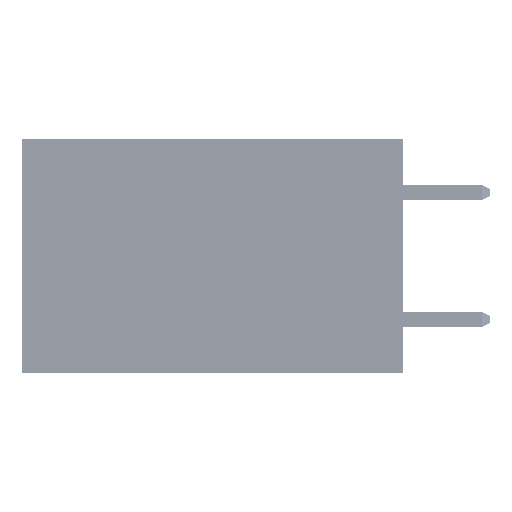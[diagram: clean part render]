
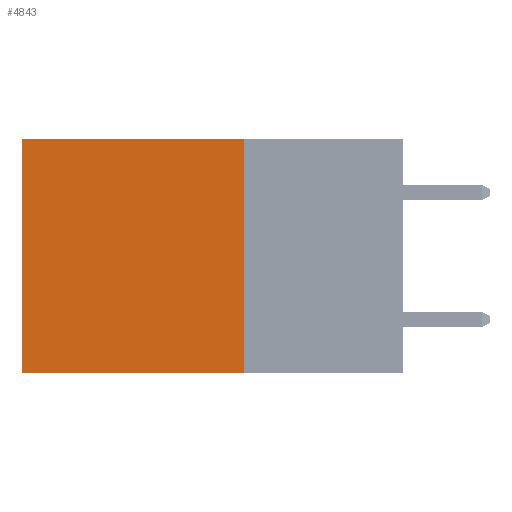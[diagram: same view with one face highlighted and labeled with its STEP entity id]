
A CAD part, left-side view. The second image highlights one B-rep face of the part: STEP entity #4843.
In plain terms, the highlighted planar face has unit normal (-1, 0, 0).
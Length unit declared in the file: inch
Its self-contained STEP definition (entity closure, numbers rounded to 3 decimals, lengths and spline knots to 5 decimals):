
#866 = ORIENTED_EDGE ( 'NONE', *, *, #38882, .F. ) ;
#1009 = CARTESIAN_POINT ( 'NONE',  ( 0.2875, 0.25, 0. ) ) ;
#1629 = CARTESIAN_POINT ( 'NONE',  ( 0.2875, 0.6, -0.37 ) ) ;
#2280 = ORIENTED_EDGE ( 'NONE', *, *, #23663, .F. ) ;
#3140 = VECTOR ( 'NONE', #40753, 39.37008 ) ;
#3284 = CARTESIAN_POINT ( 'NONE',  ( 0.2875, 0.25, 0. ) ) ;
#4843 = ADVANCED_FACE ( 'NONE', ( #8497 ), #8032, .F. ) ;
#6548 = VECTOR ( 'NONE', #10634, 39.37008 ) ;
#7323 = DIRECTION ( 'NONE',  ( 0., 0., -1. ) ) ;
#7784 = DIRECTION ( 'NONE',  ( 0., 0., -1. ) ) ;
#7798 = VECTOR ( 'NONE', #21353, 39.37008 ) ;
#8032 = PLANE ( 'NONE',  #33689 ) ;
#8497 = FACE_OUTER_BOUND ( 'NONE', #36221, .T. ) ;
#9017 = CARTESIAN_POINT ( 'NONE',  ( 0.2875, 0.25, 0. ) ) ;
#10634 = DIRECTION ( 'NONE',  ( 0., 1., 0. ) ) ;
#14505 = EDGE_CURVE ( 'NONE', #36444, #36766, #25422, .T. ) ;
#14585 = CARTESIAN_POINT ( 'NONE',  ( 0.2875, 0.6, 0. ) ) ;
#16165 = CARTESIAN_POINT ( 'NONE',  ( 0.2875, 0.25, 0. ) ) ;
#17541 = ORIENTED_EDGE ( 'NONE', *, *, #14505, .T. ) ;
#17640 = LINE ( 'NONE', #9017, #6548 ) ;
#18580 = VERTEX_POINT ( 'NONE', #16165 ) ;
#19528 = VERTEX_POINT ( 'NONE', #40727 ) ;
#21353 = DIRECTION ( 'NONE',  ( 0., 1., 0. ) ) ;
#23663 = EDGE_CURVE ( 'NONE', #19528, #36766, #36310, .T. ) ;
#25041 = LINE ( 'NONE', #3284, #3140 ) ;
#25422 = LINE ( 'NONE', #14585, #43647 ) ;
#30432 = CARTESIAN_POINT ( 'NONE',  ( 0.2875, 0.25, -0.37 ) ) ;
#30739 = EDGE_CURVE ( 'NONE', #18580, #36444, #17640, .T. ) ;
#33689 = AXIS2_PLACEMENT_3D ( 'NONE', #1009, #37756, #7784 ) ;
#36221 = EDGE_LOOP ( 'NONE', ( #17541, #2280, #866, #47207 ) ) ;
#36310 = LINE ( 'NONE', #30432, #7798 ) ;
#36444 = VERTEX_POINT ( 'NONE', #40327 ) ;
#36766 = VERTEX_POINT ( 'NONE', #1629 ) ;
#37756 = DIRECTION ( 'NONE',  ( 1., 0., 0. ) ) ;
#38882 = EDGE_CURVE ( 'NONE', #18580, #19528, #25041, .T. ) ;
#40327 = CARTESIAN_POINT ( 'NONE',  ( 0.2875, 0.6, 0. ) ) ;
#40727 = CARTESIAN_POINT ( 'NONE',  ( 0.2875, 0.25, -0.37 ) ) ;
#40753 = DIRECTION ( 'NONE',  ( 0., 0., -1. ) ) ;
#43647 = VECTOR ( 'NONE', #7323, 39.37008 ) ;
#47207 = ORIENTED_EDGE ( 'NONE', *, *, #30739, .T. ) ;
